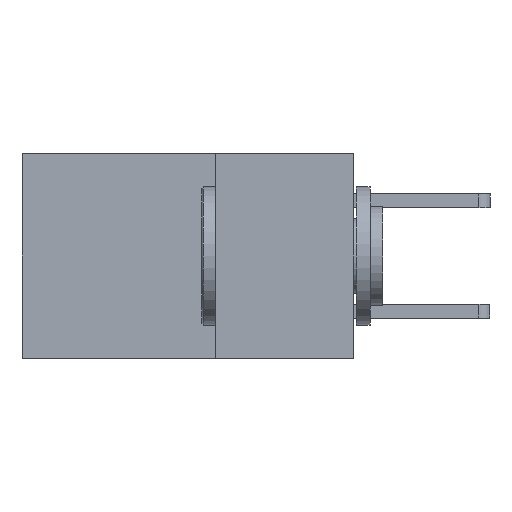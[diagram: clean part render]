
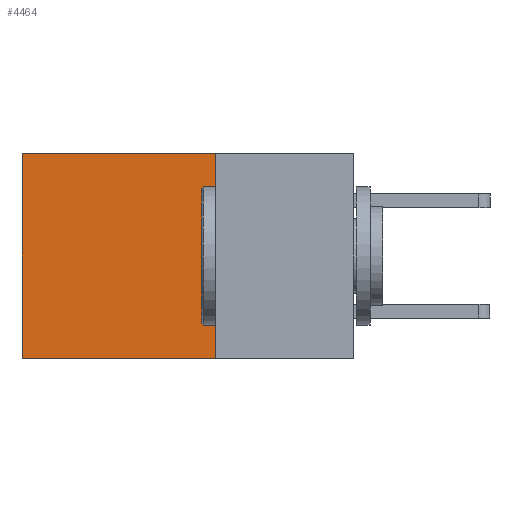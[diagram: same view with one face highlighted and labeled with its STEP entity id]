
A CAD part, left-side view. The second image highlights one B-rep face of the part: STEP entity #4464.
In plain terms, the highlighted planar face has unit normal (-1, 0, 0).
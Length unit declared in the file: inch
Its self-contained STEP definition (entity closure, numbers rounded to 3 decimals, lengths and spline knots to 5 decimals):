
#541 = VERTEX_POINT ( 'NONE', #2838 ) ;
#665 = EDGE_CURVE ( 'NONE', #5255, #965, #8557, .T. ) ;
#910 = CARTESIAN_POINT ( 'NONE',  ( 0.2875, 0.25, 0. ) ) ;
#965 = VERTEX_POINT ( 'NONE', #1354 ) ;
#1354 = CARTESIAN_POINT ( 'NONE',  ( 0.2875, 0.25, -0.37 ) ) ;
#1357 = ORIENTED_EDGE ( 'NONE', *, *, #8339, .T. ) ;
#1483 = DIRECTION ( 'NONE',  ( 1., 0., 0. ) ) ;
#1757 = CARTESIAN_POINT ( 'NONE',  ( 0.2875, 0.25, -0.37 ) ) ;
#2523 = LINE ( 'NONE', #910, #4200 ) ;
#2625 = CARTESIAN_POINT ( 'NONE',  ( 0.2875, 0.6, 0. ) ) ;
#2838 = CARTESIAN_POINT ( 'NONE',  ( 0.2875, 0.6, 0. ) ) ;
#3160 = ORIENTED_EDGE ( 'NONE', *, *, #7083, .T. ) ;
#3182 = VECTOR ( 'NONE', #5953, 39.37008 ) ;
#3335 = CARTESIAN_POINT ( 'NONE',  ( 0.2875, 0.25, 0. ) ) ;
#3381 = EDGE_CURVE ( 'NONE', #965, #5053, #5064, .T. ) ;
#3869 = ORIENTED_EDGE ( 'NONE', *, *, #665, .F. ) ;
#4144 = DIRECTION ( 'NONE',  ( 0., 0., -1. ) ) ;
#4200 = VECTOR ( 'NONE', #10567, 39.37008 ) ;
#4217 = CARTESIAN_POINT ( 'NONE',  ( 0.2875, 0.6, -0.37 ) ) ;
#4349 = CARTESIAN_POINT ( 'NONE',  ( 0.2875, 0.25, 0. ) ) ;
#4464 = ADVANCED_FACE ( 'NONE', ( #10710 ), #6756, .F. ) ;
#5053 = VERTEX_POINT ( 'NONE', #4217 ) ;
#5064 = LINE ( 'NONE', #1757, #3182 ) ;
#5255 = VERTEX_POINT ( 'NONE', #4349 ) ;
#5953 = DIRECTION ( 'NONE',  ( 0., 1., 0. ) ) ;
#6756 = PLANE ( 'NONE',  #9303 ) ;
#7083 = EDGE_CURVE ( 'NONE', #541, #5053, #10548, .T. ) ;
#7386 = ORIENTED_EDGE ( 'NONE', *, *, #3381, .F. ) ;
#7475 = DIRECTION ( 'NONE',  ( 0., 0., -1. ) ) ;
#7716 = VECTOR ( 'NONE', #7475, 39.37008 ) ;
#8339 = EDGE_CURVE ( 'NONE', #5255, #541, #2523, .T. ) ;
#8557 = LINE ( 'NONE', #10464, #10920 ) ;
#9303 = AXIS2_PLACEMENT_3D ( 'NONE', #3335, #1483, #4144 ) ;
#10341 = EDGE_LOOP ( 'NONE', ( #3160, #7386, #3869, #1357 ) ) ;
#10464 = CARTESIAN_POINT ( 'NONE',  ( 0.2875, 0.25, 0. ) ) ;
#10520 = DIRECTION ( 'NONE',  ( 0., 0., -1. ) ) ;
#10548 = LINE ( 'NONE', #2625, #7716 ) ;
#10567 = DIRECTION ( 'NONE',  ( 0., 1., 0. ) ) ;
#10710 = FACE_OUTER_BOUND ( 'NONE', #10341, .T. ) ;
#10920 = VECTOR ( 'NONE', #10520, 39.37008 ) ;
